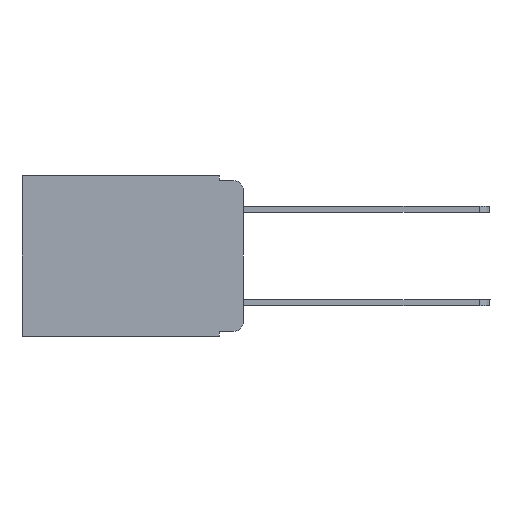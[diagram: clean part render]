
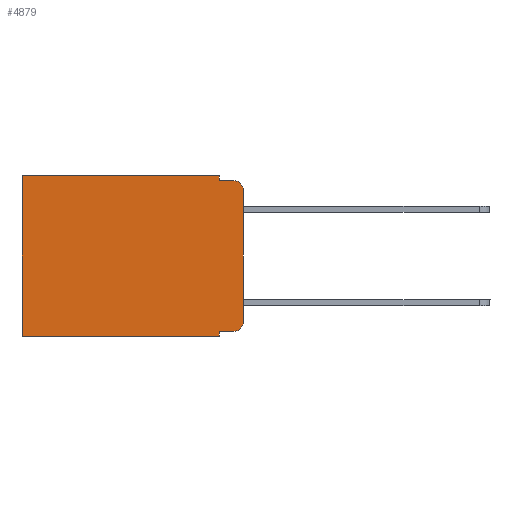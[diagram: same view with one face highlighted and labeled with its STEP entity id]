
A CAD part, left-side view. The second image highlights one B-rep face of the part: STEP entity #4879.
In plain terms, the highlighted planar face has unit normal (-1, 0, 0).
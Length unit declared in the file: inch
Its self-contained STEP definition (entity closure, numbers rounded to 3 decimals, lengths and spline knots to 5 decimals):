
#2 = DIRECTION ( 'NONE',  ( -1., 0., 0. ) ) ;
#253 = DIRECTION ( 'NONE',  ( 0., 0., -1. ) ) ;
#427 = ORIENTED_EDGE ( 'NONE', *, *, #4054, .T. ) ;
#441 = ORIENTED_EDGE ( 'NONE', *, *, #12457, .F. ) ;
#750 = VERTEX_POINT ( 'NONE', #1980 ) ;
#802 = VECTOR ( 'NONE', #10090, 39.37008 ) ;
#993 = CIRCLE ( 'NONE', #5686, 0.02 ) ;
#1001 = EDGE_LOOP ( 'NONE', ( #441, #3512, #8978, #1748, #12319, #2741, #7097, #6874, #427, #10998 ) ) ;
#1277 = PLANE ( 'NONE',  #5890 ) ;
#1321 = DIRECTION ( 'NONE',  ( 0., -1., 0. ) ) ;
#1492 = DIRECTION ( 'NONE',  ( 0., 0., -1. ) ) ;
#1581 = CARTESIAN_POINT ( 'NONE',  ( 0.298, 0.051, 0. ) ) ;
#1748 = ORIENTED_EDGE ( 'NONE', *, *, #9681, .F. ) ;
#1980 = CARTESIAN_POINT ( 'NONE',  ( 0.298, 0.051, -0.343 ) ) ;
#2293 = VERTEX_POINT ( 'NONE', #6328 ) ;
#2320 = EDGE_CURVE ( 'NONE', #2455, #6848, #993, .T. ) ;
#2455 = VERTEX_POINT ( 'NONE', #9984 ) ;
#2536 = LINE ( 'NONE', #10997, #11050 ) ;
#2741 = ORIENTED_EDGE ( 'NONE', *, *, #10648, .T. ) ;
#2803 = VECTOR ( 'NONE', #1492, 39.37008 ) ;
#2843 = VERTEX_POINT ( 'NONE', #1581 ) ;
#3225 = LINE ( 'NONE', #12243, #802 ) ;
#3306 = LINE ( 'NONE', #4611, #2803 ) ;
#3512 = ORIENTED_EDGE ( 'NONE', *, *, #2320, .T. ) ;
#3639 = DIRECTION ( 'NONE',  ( -1., 0., 0. ) ) ;
#4054 = EDGE_CURVE ( 'NONE', #4191, #11901, #10937, .T. ) ;
#4191 = VERTEX_POINT ( 'NONE', #12610 ) ;
#4501 = EDGE_CURVE ( 'NONE', #2293, #6848, #3225, .T. ) ;
#4611 = CARTESIAN_POINT ( 'NONE',  ( 0.298, 0., 0. ) ) ;
#4758 = CARTESIAN_POINT ( 'NONE',  ( 0.298, 0.02, -0.03 ) ) ;
#4876 = DIRECTION ( 'NONE',  ( 0., 0., -1. ) ) ;
#4879 = ADVANCED_FACE ( 'NONE', ( #6617 ), #1277, .F. ) ;
#4910 = VECTOR ( 'NONE', #11708, 39.37008 ) ;
#5473 = LINE ( 'NONE', #8163, #12027 ) ;
#5686 = AXIS2_PLACEMENT_3D ( 'NONE', #4758, #3639, #8940 ) ;
#5845 = CARTESIAN_POINT ( 'NONE',  ( 0.298, 0.02, -0.01 ) ) ;
#5890 = AXIS2_PLACEMENT_3D ( 'NONE', #8362, #12525, #253 ) ;
#6103 = CARTESIAN_POINT ( 'NONE',  ( 0.298, 0.051, -0.333 ) ) ;
#6328 = CARTESIAN_POINT ( 'NONE',  ( 0.298, 0.051, -0.01 ) ) ;
#6538 = VERTEX_POINT ( 'NONE', #11265 ) ;
#6617 = FACE_OUTER_BOUND ( 'NONE', #1001, .T. ) ;
#6707 = CIRCLE ( 'NONE', #9799, 0.02 ) ;
#6848 = VERTEX_POINT ( 'NONE', #5845 ) ;
#6874 = ORIENTED_EDGE ( 'NONE', *, *, #8404, .F. ) ;
#6987 = VECTOR ( 'NONE', #10120, 39.37008 ) ;
#7097 = ORIENTED_EDGE ( 'NONE', *, *, #12519, .F. ) ;
#7974 = DIRECTION ( 'NONE',  ( 0., 1., 0. ) ) ;
#8163 = CARTESIAN_POINT ( 'NONE',  ( 0.298, 0., 0. ) ) ;
#8362 = CARTESIAN_POINT ( 'NONE',  ( 0.298, 0., 0. ) ) ;
#8404 = EDGE_CURVE ( 'NONE', #4191, #750, #9404, .T. ) ;
#8940 = DIRECTION ( 'NONE',  ( 0., 0., -1. ) ) ;
#8966 = CARTESIAN_POINT ( 'NONE',  ( 0.298, 0.473, -0.343 ) ) ;
#8978 = ORIENTED_EDGE ( 'NONE', *, *, #4501, .F. ) ;
#8981 = CARTESIAN_POINT ( 'NONE',  ( 0.298, 0.02, -0.333 ) ) ;
#9404 = LINE ( 'NONE', #12697, #4910 ) ;
#9489 = CARTESIAN_POINT ( 'NONE',  ( 0.298, 0.473, 0. ) ) ;
#9681 = EDGE_CURVE ( 'NONE', #2843, #2293, #9688, .T. ) ;
#9688 = LINE ( 'NONE', #12157, #6987 ) ;
#9720 = VECTOR ( 'NONE', #7974, 39.37008 ) ;
#9799 = AXIS2_PLACEMENT_3D ( 'NONE', #10292, #2, #11339 ) ;
#9984 = CARTESIAN_POINT ( 'NONE',  ( 0.298, 0., -0.03 ) ) ;
#10090 = DIRECTION ( 'NONE',  ( 0., -1., 0. ) ) ;
#10120 = DIRECTION ( 'NONE',  ( 0., 0., -1. ) ) ;
#10292 = CARTESIAN_POINT ( 'NONE',  ( 0.298, 0.02, -0.313 ) ) ;
#10298 = EDGE_CURVE ( 'NONE', #2843, #10378, #5473, .T. ) ;
#10378 = VERTEX_POINT ( 'NONE', #9489 ) ;
#10648 = EDGE_CURVE ( 'NONE', #10378, #12627, #2536, .T. ) ;
#10937 = LINE ( 'NONE', #6103, #13019 ) ;
#10997 = CARTESIAN_POINT ( 'NONE',  ( 0.298, 0.473, 0. ) ) ;
#10998 = ORIENTED_EDGE ( 'NONE', *, *, #12143, .T. ) ;
#11050 = VECTOR ( 'NONE', #4876, 39.37008 ) ;
#11265 = CARTESIAN_POINT ( 'NONE',  ( 0.298, 0., -0.313 ) ) ;
#11285 = DIRECTION ( 'NONE',  ( 0., 1., 0. ) ) ;
#11339 = DIRECTION ( 'NONE',  ( 0., 0., -1. ) ) ;
#11708 = DIRECTION ( 'NONE',  ( 0., 0., -1. ) ) ;
#11901 = VERTEX_POINT ( 'NONE', #8981 ) ;
#12027 = VECTOR ( 'NONE', #11285, 39.37008 ) ;
#12143 = EDGE_CURVE ( 'NONE', #11901, #6538, #6707, .T. ) ;
#12157 = CARTESIAN_POINT ( 'NONE',  ( 0.298, 0.051, 0. ) ) ;
#12243 = CARTESIAN_POINT ( 'NONE',  ( 0.298, 0.051, -0.01 ) ) ;
#12319 = ORIENTED_EDGE ( 'NONE', *, *, #10298, .T. ) ;
#12449 = LINE ( 'NONE', #12842, #9720 ) ;
#12457 = EDGE_CURVE ( 'NONE', #2455, #6538, #3306, .T. ) ;
#12519 = EDGE_CURVE ( 'NONE', #750, #12627, #12449, .T. ) ;
#12525 = DIRECTION ( 'NONE',  ( 1., 0., 0. ) ) ;
#12610 = CARTESIAN_POINT ( 'NONE',  ( 0.298, 0.051, -0.333 ) ) ;
#12627 = VERTEX_POINT ( 'NONE', #8966 ) ;
#12697 = CARTESIAN_POINT ( 'NONE',  ( 0.298, 0.051, 0. ) ) ;
#12842 = CARTESIAN_POINT ( 'NONE',  ( 0.298, 0., -0.343 ) ) ;
#13019 = VECTOR ( 'NONE', #1321, 39.37008 ) ;
